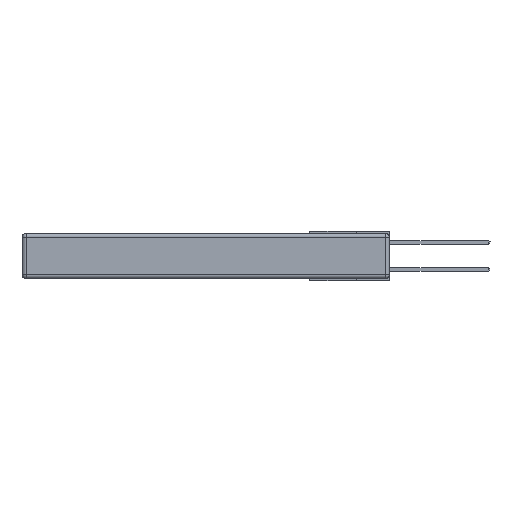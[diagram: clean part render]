
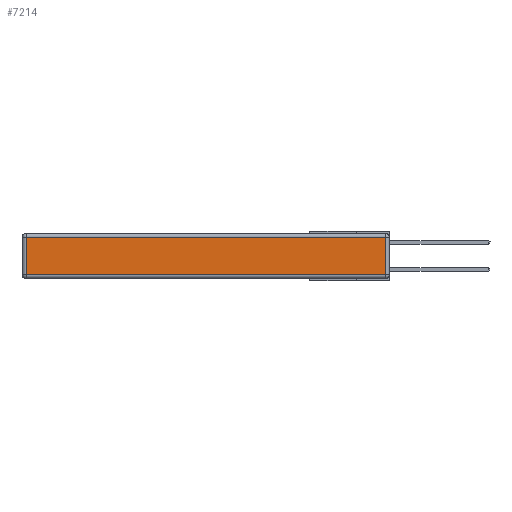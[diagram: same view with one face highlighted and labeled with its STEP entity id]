
A CAD part, left-side view. The second image highlights one B-rep face of the part: STEP entity #7214.
In plain terms, the highlighted planar face has unit normal (-1, 0, 0).
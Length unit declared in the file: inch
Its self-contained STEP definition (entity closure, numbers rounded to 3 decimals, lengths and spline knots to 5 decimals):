
#37 = CARTESIAN_POINT ( 'NONE',  ( 0., 0., -0.343 ) ) ;
#451 = VECTOR ( 'NONE', #13164, 39.37008 ) ;
#1964 = LINE ( 'NONE', #17552, #8969 ) ;
#1979 = DIRECTION ( 'NONE',  ( 0., 0., 1. ) ) ;
#3492 = DIRECTION ( 'NONE',  ( 0., 1., 0. ) ) ;
#4297 = DIRECTION ( 'NONE',  ( 0., 0., 1. ) ) ;
#4436 = LINE ( 'NONE', #18791, #451 ) ;
#4513 = VERTEX_POINT ( 'NONE', #15133 ) ;
#4547 = VERTEX_POINT ( 'NONE', #6606 ) ;
#4888 = EDGE_CURVE ( 'NONE', #13635, #4547, #1964, .T. ) ;
#5015 = LINE ( 'NONE', #6584, #10817 ) ;
#5472 = VERTEX_POINT ( 'NONE', #13586 ) ;
#6584 = CARTESIAN_POINT ( 'NONE',  ( 0., 2.75, -0.03 ) ) ;
#6606 = CARTESIAN_POINT ( 'NONE',  ( 0., 2.72, -0.313 ) ) ;
#7214 = ADVANCED_FACE ( 'NONE', ( #16760 ), #15101, .T. ) ;
#7264 = DIRECTION ( 'NONE',  ( 0., 0., -1. ) ) ;
#7517 = AXIS2_PLACEMENT_3D ( 'NONE', #37, #10453, #1979 ) ;
#7604 = EDGE_CURVE ( 'NONE', #4547, #5472, #4436, .T. ) ;
#7939 = VECTOR ( 'NONE', #4297, 39.37008 ) ;
#8161 = ORIENTED_EDGE ( 'NONE', *, *, #16148, .T. ) ;
#8507 = EDGE_CURVE ( 'NONE', #5472, #4513, #17424, .T. ) ;
#8835 = ORIENTED_EDGE ( 'NONE', *, *, #8507, .T. ) ;
#8969 = VECTOR ( 'NONE', #7264, 39.37008 ) ;
#10453 = DIRECTION ( 'NONE',  ( -1., 0., 0. ) ) ;
#10817 = VECTOR ( 'NONE', #3492, 39.37008 ) ;
#13164 = DIRECTION ( 'NONE',  ( 0., -1., 0. ) ) ;
#13586 = CARTESIAN_POINT ( 'NONE',  ( 0., 0.03, -0.313 ) ) ;
#13635 = VERTEX_POINT ( 'NONE', #15788 ) ;
#14362 = EDGE_LOOP ( 'NONE', ( #17468, #8835, #8161, #17289 ) ) ;
#15101 = PLANE ( 'NONE',  #7517 ) ;
#15133 = CARTESIAN_POINT ( 'NONE',  ( 0., 0.03, -0.03 ) ) ;
#15788 = CARTESIAN_POINT ( 'NONE',  ( 0., 2.72, -0.03 ) ) ;
#16148 = EDGE_CURVE ( 'NONE', #4513, #13635, #5015, .T. ) ;
#16760 = FACE_OUTER_BOUND ( 'NONE', #14362, .T. ) ;
#17289 = ORIENTED_EDGE ( 'NONE', *, *, #4888, .T. ) ;
#17424 = LINE ( 'NONE', #18123, #7939 ) ;
#17468 = ORIENTED_EDGE ( 'NONE', *, *, #7604, .T. ) ;
#17552 = CARTESIAN_POINT ( 'NONE',  ( 0., 2.72, -0.343 ) ) ;
#18123 = CARTESIAN_POINT ( 'NONE',  ( 0., 0.03, -0.343 ) ) ;
#18791 = CARTESIAN_POINT ( 'NONE',  ( 0., 0., -0.313 ) ) ;
